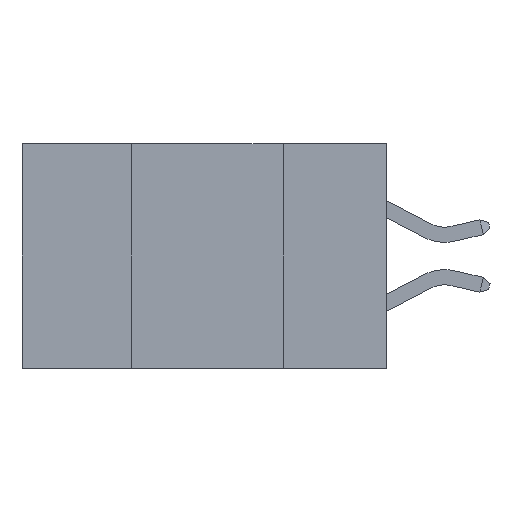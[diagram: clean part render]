
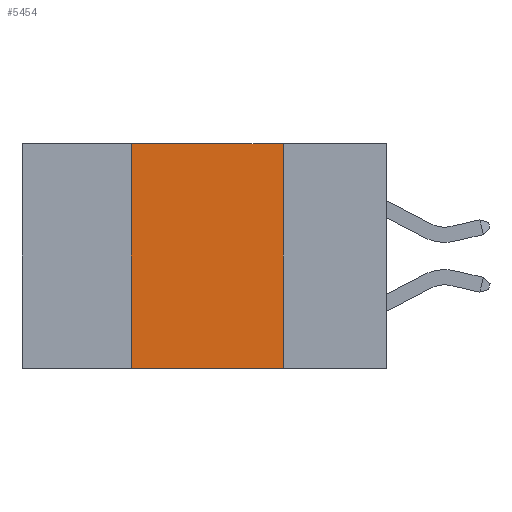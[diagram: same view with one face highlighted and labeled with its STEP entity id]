
A CAD part, left-side view. The second image highlights one B-rep face of the part: STEP entity #5454.
In plain terms, the highlighted planar face has unit normal (-1, 0, 0).
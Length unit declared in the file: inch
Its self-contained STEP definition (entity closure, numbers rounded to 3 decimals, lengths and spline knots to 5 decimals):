
#256 = ORIENTED_EDGE ( 'NONE', *, *, #14414, .F. ) ;
#1270 = LINE ( 'NONE', #2013, #16444 ) ;
#1419 = PLANE ( 'NONE',  #7734 ) ;
#1797 = EDGE_CURVE ( 'NONE', #14689, #4400, #11675, .T. ) ;
#2013 = CARTESIAN_POINT ( 'NONE',  ( 0., 0.6, 0. ) ) ;
#2127 = VECTOR ( 'NONE', #11545, 39.37008 ) ;
#2672 = DIRECTION ( 'NONE',  ( 0., 0., 1. ) ) ;
#2693 = VECTOR ( 'NONE', #6453, 39.37008 ) ;
#3087 = CARTESIAN_POINT ( 'NONE',  ( 0., 0.42, -0.37 ) ) ;
#3215 = VERTEX_POINT ( 'NONE', #13859 ) ;
#3275 = DIRECTION ( 'NONE',  ( 0., -1., 0. ) ) ;
#3445 = EDGE_CURVE ( 'NONE', #17191, #4400, #17237, .T. ) ;
#3789 = ORIENTED_EDGE ( 'NONE', *, *, #3445, .T. ) ;
#4400 = VERTEX_POINT ( 'NONE', #4633 ) ;
#4633 = CARTESIAN_POINT ( 'NONE',  ( 0., 0.17, -0.37 ) ) ;
#5454 = ADVANCED_FACE ( 'NONE', ( #6156 ), #1419, .F. ) ;
#6156 = FACE_OUTER_BOUND ( 'NONE', #9069, .T. ) ;
#6435 = ORIENTED_EDGE ( 'NONE', *, *, #9942, .F. ) ;
#6453 = DIRECTION ( 'NONE',  ( 0., -1., 0. ) ) ;
#7424 = CARTESIAN_POINT ( 'NONE',  ( 0., 0.17, 0. ) ) ;
#7734 = AXIS2_PLACEMENT_3D ( 'NONE', #12390, #14812, #16681 ) ;
#8303 = ORIENTED_EDGE ( 'NONE', *, *, #1797, .F. ) ;
#8477 = CARTESIAN_POINT ( 'NONE',  ( 0., 0.42, 0. ) ) ;
#9069 = EDGE_LOOP ( 'NONE', ( #8303, #256, #6435, #3789 ) ) ;
#9942 = EDGE_CURVE ( 'NONE', #17191, #3215, #17647, .T. ) ;
#11545 = DIRECTION ( 'NONE',  ( 0., 0., -1. ) ) ;
#11658 = CARTESIAN_POINT ( 'NONE',  ( 0., 0.17, 0. ) ) ;
#11675 = LINE ( 'NONE', #11658, #2127 ) ;
#12390 = CARTESIAN_POINT ( 'NONE',  ( 0., 0.6, 0. ) ) ;
#13859 = CARTESIAN_POINT ( 'NONE',  ( 0., 0.42, 0. ) ) ;
#14414 = EDGE_CURVE ( 'NONE', #3215, #14689, #1270, .T. ) ;
#14689 = VERTEX_POINT ( 'NONE', #7424 ) ;
#14812 = DIRECTION ( 'NONE',  ( 1., 0., 0. ) ) ;
#16233 = CARTESIAN_POINT ( 'NONE',  ( 0., 0.6, -0.37 ) ) ;
#16444 = VECTOR ( 'NONE', #3275, 39.37008 ) ;
#16681 = DIRECTION ( 'NONE',  ( 0., 0., -1. ) ) ;
#17191 = VERTEX_POINT ( 'NONE', #3087 ) ;
#17214 = VECTOR ( 'NONE', #2672, 39.37008 ) ;
#17237 = LINE ( 'NONE', #16233, #2693 ) ;
#17647 = LINE ( 'NONE', #8477, #17214 ) ;
